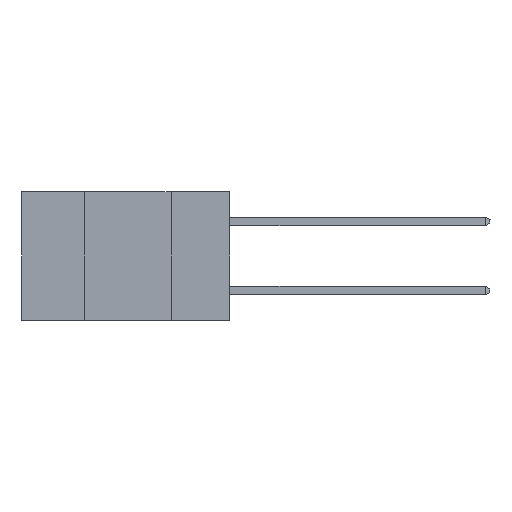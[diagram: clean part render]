
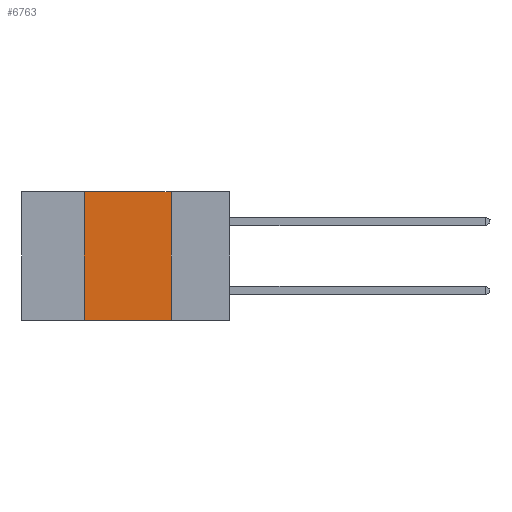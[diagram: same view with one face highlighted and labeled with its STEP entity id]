
A CAD part, left-side view. The second image highlights one B-rep face of the part: STEP entity #6763.
In plain terms, the highlighted planar face has unit normal (-1, 0, 0).
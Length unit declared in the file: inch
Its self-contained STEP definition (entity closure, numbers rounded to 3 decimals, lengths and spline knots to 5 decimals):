
#1380 = VERTEX_POINT ( 'NONE', #16324 ) ;
#2092 = ORIENTED_EDGE ( 'NONE', *, *, #12329, .T. ) ;
#2619 = LINE ( 'NONE', #16645, #19452 ) ;
#2963 = DIRECTION ( 'NONE',  ( 0., 0., -1. ) ) ;
#3731 = DIRECTION ( 'NONE',  ( 0., 0., 1. ) ) ;
#3741 = VECTOR ( 'NONE', #9664, 39.37008 ) ;
#4097 = VECTOR ( 'NONE', #20259, 39.37008 ) ;
#5486 = EDGE_LOOP ( 'NONE', ( #19605, #16381, #16808, #2092 ) ) ;
#5912 = VERTEX_POINT ( 'NONE', #6469 ) ;
#6007 = VECTOR ( 'NONE', #6938, 39.37008 ) ;
#6218 = CARTESIAN_POINT ( 'NONE',  ( 0., 0.6, 0. ) ) ;
#6469 = CARTESIAN_POINT ( 'NONE',  ( 0., 0.17, -0.37 ) ) ;
#6763 = ADVANCED_FACE ( 'NONE', ( #17845 ), #15833, .F. ) ;
#6938 = DIRECTION ( 'NONE',  ( 0., -1., 0. ) ) ;
#8288 = VERTEX_POINT ( 'NONE', #15826 ) ;
#8993 = EDGE_CURVE ( 'NONE', #18491, #1380, #2619, .T. ) ;
#9454 = DIRECTION ( 'NONE',  ( 1., 0., 0. ) ) ;
#9664 = DIRECTION ( 'NONE',  ( 0., -1., 0. ) ) ;
#9948 = CARTESIAN_POINT ( 'NONE',  ( 0., 0.6, 0. ) ) ;
#10027 = LINE ( 'NONE', #18459, #6007 ) ;
#12329 = EDGE_CURVE ( 'NONE', #18491, #5912, #10027, .T. ) ;
#12643 = LINE ( 'NONE', #15529, #4097 ) ;
#13655 = EDGE_CURVE ( 'NONE', #8288, #5912, #12643, .T. ) ;
#15529 = CARTESIAN_POINT ( 'NONE',  ( 0., 0.17, 0. ) ) ;
#15826 = CARTESIAN_POINT ( 'NONE',  ( 0., 0.17, 0. ) ) ;
#15833 = PLANE ( 'NONE',  #20786 ) ;
#16324 = CARTESIAN_POINT ( 'NONE',  ( 0., 0.42, 0. ) ) ;
#16381 = ORIENTED_EDGE ( 'NONE', *, *, #19711, .F. ) ;
#16645 = CARTESIAN_POINT ( 'NONE',  ( 0., 0.42, 0. ) ) ;
#16808 = ORIENTED_EDGE ( 'NONE', *, *, #8993, .F. ) ;
#17845 = FACE_OUTER_BOUND ( 'NONE', #5486, .T. ) ;
#18459 = CARTESIAN_POINT ( 'NONE',  ( 0., 0.6, -0.37 ) ) ;
#18491 = VERTEX_POINT ( 'NONE', #19231 ) ;
#19231 = CARTESIAN_POINT ( 'NONE',  ( 0., 0.42, -0.37 ) ) ;
#19452 = VECTOR ( 'NONE', #3731, 39.37008 ) ;
#19605 = ORIENTED_EDGE ( 'NONE', *, *, #13655, .F. ) ;
#19711 = EDGE_CURVE ( 'NONE', #1380, #8288, #19809, .T. ) ;
#19809 = LINE ( 'NONE', #9948, #3741 ) ;
#20259 = DIRECTION ( 'NONE',  ( 0., 0., -1. ) ) ;
#20786 = AXIS2_PLACEMENT_3D ( 'NONE', #6218, #9454, #2963 ) ;
